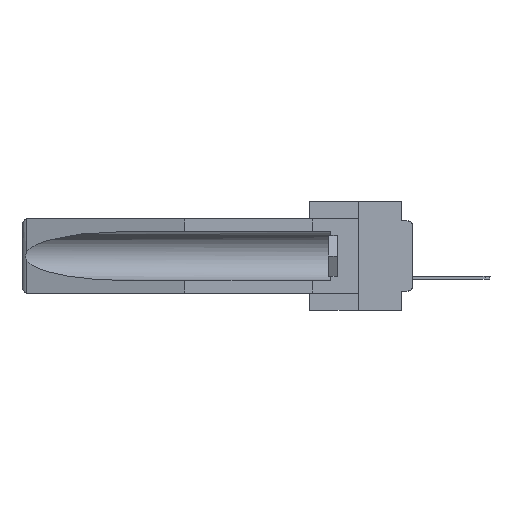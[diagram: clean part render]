
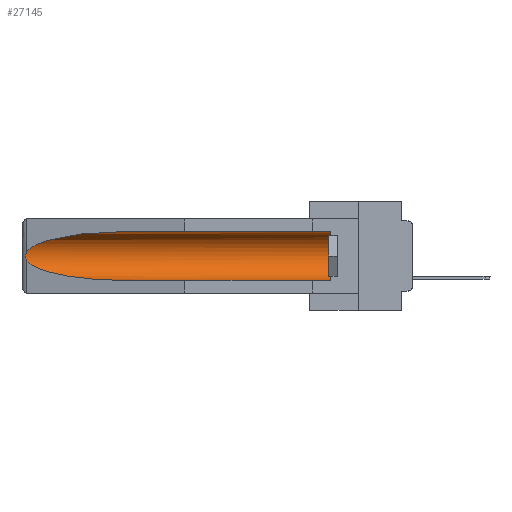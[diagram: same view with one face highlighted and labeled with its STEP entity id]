
A CAD part, left-side view. The second image highlights one B-rep face of the part: STEP entity #27145.
In plain terms, the highlighted cylindrical face has radius 2.857 mm (diameter 5.715 mm), a partial arc.
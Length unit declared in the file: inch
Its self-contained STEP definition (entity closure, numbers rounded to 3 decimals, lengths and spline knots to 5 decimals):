
#63 = CARTESIAN_POINT ( 'NONE',  ( 0.155, -0.30754, -0.059 ) ) ;
#445 = DIRECTION ( 'NONE',  ( 0., -1., 0. ) ) ;
#3293 = CARTESIAN_POINT ( 'NONE',  ( 0.155, 0.126, -0.059 ) ) ;
#3531 = CARTESIAN_POINT ( 'NONE',  ( 0.155, 1.07973, -0.284 ) ) ;
#3807 = EDGE_CURVE ( 'NONE', #27455, #14400, #14501, .T. ) ;
#4178 = VERTEX_POINT ( 'NONE', #24078 ) ;
#4414 =( BOUNDED_CURVE ( )  B_SPLINE_CURVE ( 3, ( #5011, #28783, #21706, #24051 ),
 .UNSPECIFIED., .F., .F. ) 
 B_SPLINE_CURVE_WITH_KNOTS ( ( 4, 4 ),
 ( 4.71239, 6.08839 ),
 .UNSPECIFIED. ) 
 CURVE ( )  GEOMETRIC_REPRESENTATION_ITEM ( )  RATIONAL_B_SPLINE_CURVE ( ( 1., 0.848, 0.848, 1. ) ) 
 REPRESENTATION_ITEM ( '' )  );
#4973 = CARTESIAN_POINT ( 'NONE',  ( 0.26597, 1.5296, -0.19026 ) ) ;
#5011 = CARTESIAN_POINT ( 'NONE',  ( 0.155, 1.07973, -0.059 ) ) ;
#5308 = CARTESIAN_POINT ( 'NONE',  ( 0.155, -0.30754, -0.284 ) ) ;
#5848 = DIRECTION ( 'NONE',  ( 0., 0., 1. ) ) ;
#5977 = VECTOR ( 'NONE', #27016, 39.37008 ) ;
#6166 = EDGE_CURVE ( 'NONE', #14400, #18785, #4414, .T. ) ;
#6778 = CARTESIAN_POINT ( 'NONE',  ( 0.26537, 1.52718, -0.19328 ) ) ;
#7022 = CARTESIAN_POINT ( 'NONE',  ( 0.2673, 1.53269, -0.17917 ) ) ;
#7174 = CARTESIAN_POINT ( 'NONE',  ( 0.26654, 1.53092, -0.15636 ) ) ;
#7437 = DIRECTION ( 'NONE',  ( 0., 1., 0. ) ) ;
#8804 = CIRCLE ( 'NONE', #18872, 0.1125 ) ;
#9381 = CARTESIAN_POINT ( 'NONE',  ( 0.2673, 1.5327, -0.16383 ) ) ;
#9872 = ORIENTED_EDGE ( 'NONE', *, *, #22025, .F. ) ;
#9978 = VERTEX_POINT ( 'NONE', #6778 ) ;
#10730 = CARTESIAN_POINT ( 'NONE',  ( 0.155, -0.30754, -0.1715 ) ) ;
#11908 = CARTESIAN_POINT ( 'NONE',  ( 0.26597, 1.52961, -0.15275 ) ) ;
#12020 = EDGE_CURVE ( 'NONE', #9978, #28450, #28946, .T. ) ;
#13390 = ORIENTED_EDGE ( 'NONE', *, *, #15707, .T. ) ;
#13877 = ORIENTED_EDGE ( 'NONE', *, *, #12020, .T. ) ;
#14094 = ORIENTED_EDGE ( 'NONE', *, *, #3807, .T. ) ;
#14248 = CARTESIAN_POINT ( 'NONE',  ( 0.25451, 1.48313, -0.24835 ) ) ;
#14276 = EDGE_LOOP ( 'NONE', ( #21362, #13390, #13877, #9872, #27966, #14094 ) ) ;
#14400 = VERTEX_POINT ( 'NONE', #25145 ) ;
#14501 = LINE ( 'NONE', #63, #23622 ) ;
#14844 = CARTESIAN_POINT ( 'NONE',  ( 0.26537, 1.52718, -0.14972 ) ) ;
#15707 = EDGE_CURVE ( 'NONE', #18785, #9978, #18357, .T. ) ;
#16464 = CARTESIAN_POINT ( 'NONE',  ( 0.26537, 1.52718, -0.14972 ) ) ;
#16614 = CARTESIAN_POINT ( 'NONE',  ( 0.2675, 1.53308, -0.17534 ) ) ;
#16772 = CARTESIAN_POINT ( 'NONE',  ( 0.26537, 1.52718, -0.19328 ) ) ;
#17261 = LINE ( 'NONE', #5308, #5977 ) ;
#18357 = B_SPLINE_CURVE_WITH_KNOTS ( 'NONE', 3,
 ( #16464, #11908, #7174, #9381, #31104, #16614, #7022, #21509, #4973, #16772 ),
 .UNSPECIFIED., .F., .F.,
 ( 4, 2, 2, 2, 4 ),
 ( 0., 0.00029, 0.00058, 0.00087, 0.00117 ),
 .UNSPECIFIED. ) ;
#18785 = VERTEX_POINT ( 'NONE', #14844 ) ;
#18835 = CARTESIAN_POINT ( 'NONE',  ( 0.155, 1.07973, -0.284 ) ) ;
#18872 = AXIS2_PLACEMENT_3D ( 'NONE', #21699, #445, #26881 ) ;
#20236 = EDGE_CURVE ( 'NONE', #4178, #27455, #8804, .T. ) ;
#20477 = FACE_OUTER_BOUND ( 'NONE', #14276, .T. ) ;
#21362 = ORIENTED_EDGE ( 'NONE', *, *, #6166, .T. ) ;
#21509 = CARTESIAN_POINT ( 'NONE',  ( 0.26655, 1.53094, -0.18657 ) ) ;
#21699 = CARTESIAN_POINT ( 'NONE',  ( 0.155, 0.126, -0.1715 ) ) ;
#21706 = CARTESIAN_POINT ( 'NONE',  ( 0.25451, 1.48313, -0.09465 ) ) ;
#22025 = EDGE_CURVE ( 'NONE', #4178, #28450, #17261, .T. ) ;
#23622 = VECTOR ( 'NONE', #7437, 39.37008 ) ;
#24051 = CARTESIAN_POINT ( 'NONE',  ( 0.26537, 1.52718, -0.14972 ) ) ;
#24078 = CARTESIAN_POINT ( 'NONE',  ( 0.155, 0.126, -0.284 ) ) ;
#25145 = CARTESIAN_POINT ( 'NONE',  ( 0.155, 1.07973, -0.059 ) ) ;
#25755 = AXIS2_PLACEMENT_3D ( 'NONE', #10730, #27737, #5848 ) ;
#26881 = DIRECTION ( 'NONE',  ( 0., 0., 1. ) ) ;
#27016 = DIRECTION ( 'NONE',  ( 0., 1., 0. ) ) ;
#27145 = ADVANCED_FACE ( 'NONE', ( #20477 ), #27417, .F. ) ;
#27417 = CYLINDRICAL_SURFACE ( 'NONE', #25755, 0.1125 ) ;
#27455 = VERTEX_POINT ( 'NONE', #3293 ) ;
#27737 = DIRECTION ( 'NONE',  ( 0., 1., 0. ) ) ;
#27966 = ORIENTED_EDGE ( 'NONE', *, *, #20236, .T. ) ;
#28436 = CARTESIAN_POINT ( 'NONE',  ( 0.21114, 1.30732, -0.284 ) ) ;
#28450 = VERTEX_POINT ( 'NONE', #3531 ) ;
#28783 = CARTESIAN_POINT ( 'NONE',  ( 0.21114, 1.30732, -0.059 ) ) ;
#28946 =( BOUNDED_CURVE ( )  B_SPLINE_CURVE ( 3, ( #30479, #14248, #28436, #18835 ),
 .UNSPECIFIED., .F., .F. ) 
 B_SPLINE_CURVE_WITH_KNOTS ( ( 4, 4 ),
 ( 0.1948, 1.5708 ),
 .UNSPECIFIED. ) 
 CURVE ( )  GEOMETRIC_REPRESENTATION_ITEM ( )  RATIONAL_B_SPLINE_CURVE ( ( 1., 0.848, 0.848, 1. ) ) 
 REPRESENTATION_ITEM ( '' )  );
#30479 = CARTESIAN_POINT ( 'NONE',  ( 0.26537, 1.52718, -0.19328 ) ) ;
#31104 = CARTESIAN_POINT ( 'NONE',  ( 0.2675, 1.53308, -0.16763 ) ) ;
